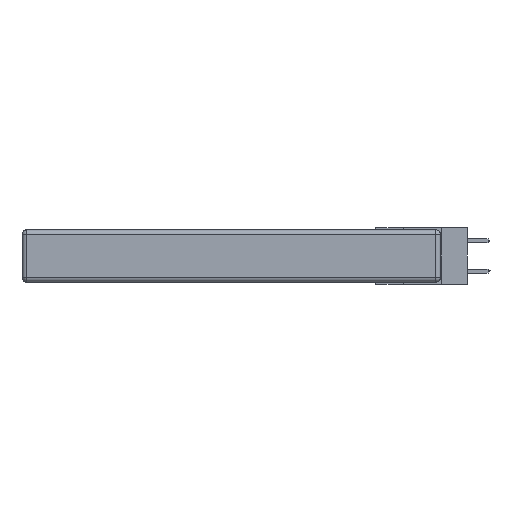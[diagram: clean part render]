
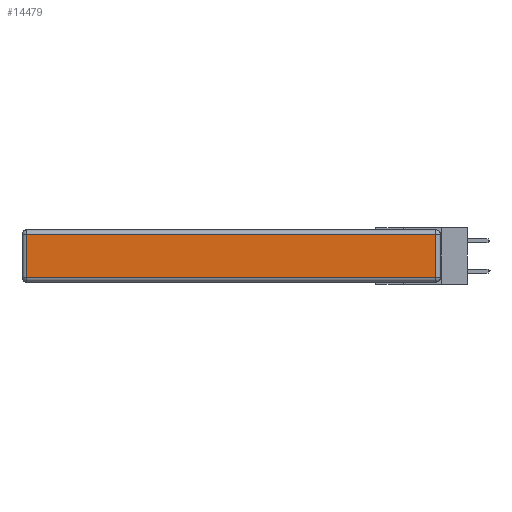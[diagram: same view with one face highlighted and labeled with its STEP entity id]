
A CAD part, left-side view. The second image highlights one B-rep face of the part: STEP entity #14479.
In plain terms, the highlighted planar face has unit normal (-1, 0, 0).
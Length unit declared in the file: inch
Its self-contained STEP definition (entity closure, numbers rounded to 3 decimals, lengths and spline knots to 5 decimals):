
#34 = CARTESIAN_POINT ( 'NONE',  ( 0., 2.72, -0.03 ) ) ;
#37 = DIRECTION ( 'NONE',  ( 0., 0., 1. ) ) ;
#346 = LINE ( 'NONE', #25565, #20899 ) ;
#1693 = ORIENTED_EDGE ( 'NONE', *, *, #17655, .T. ) ;
#5072 = VERTEX_POINT ( 'NONE', #11036 ) ;
#5687 = DIRECTION ( 'NONE',  ( 0., 1., 0. ) ) ;
#5783 = CARTESIAN_POINT ( 'NONE',  ( 0., 2.75, -0.03 ) ) ;
#7728 = CARTESIAN_POINT ( 'NONE',  ( 0., 0., -0.313 ) ) ;
#8910 = CARTESIAN_POINT ( 'NONE',  ( 0., 0.03, -0.343 ) ) ;
#9664 = DIRECTION ( 'NONE',  ( 0., -1., 0. ) ) ;
#10783 = PLANE ( 'NONE',  #12081 ) ;
#11036 = CARTESIAN_POINT ( 'NONE',  ( 0., 2.72, -0.313 ) ) ;
#11377 = VERTEX_POINT ( 'NONE', #17019 ) ;
#12081 = AXIS2_PLACEMENT_3D ( 'NONE', #24100, #13170, #37 ) ;
#12638 = VECTOR ( 'NONE', #9664, 39.37008 ) ;
#13128 = DIRECTION ( 'NONE',  ( 0., 0., 1. ) ) ;
#13170 = DIRECTION ( 'NONE',  ( -1., 0., 0. ) ) ;
#14479 = ADVANCED_FACE ( 'NONE', ( #22156 ), #10783, .T. ) ;
#14564 = ORIENTED_EDGE ( 'NONE', *, *, #26897, .T. ) ;
#15314 = EDGE_CURVE ( 'NONE', #11377, #20907, #17963, .T. ) ;
#15603 = VECTOR ( 'NONE', #5687, 39.37008 ) ;
#17019 = CARTESIAN_POINT ( 'NONE',  ( 0., 0.03, -0.03 ) ) ;
#17655 = EDGE_CURVE ( 'NONE', #20907, #5072, #346, .T. ) ;
#17670 = ORIENTED_EDGE ( 'NONE', *, *, #15314, .T. ) ;
#17800 = ORIENTED_EDGE ( 'NONE', *, *, #22877, .T. ) ;
#17963 = LINE ( 'NONE', #5783, #15603 ) ;
#18125 = LINE ( 'NONE', #8910, #22605 ) ;
#18182 = LINE ( 'NONE', #7728, #12638 ) ;
#19935 = VERTEX_POINT ( 'NONE', #27372 ) ;
#20899 = VECTOR ( 'NONE', #27961, 39.37008 ) ;
#20907 = VERTEX_POINT ( 'NONE', #34 ) ;
#22156 = FACE_OUTER_BOUND ( 'NONE', #26323, .T. ) ;
#22605 = VECTOR ( 'NONE', #13128, 39.37008 ) ;
#22877 = EDGE_CURVE ( 'NONE', #19935, #11377, #18125, .T. ) ;
#24100 = CARTESIAN_POINT ( 'NONE',  ( 0., 0., -0.343 ) ) ;
#25565 = CARTESIAN_POINT ( 'NONE',  ( 0., 2.72, -0.343 ) ) ;
#26323 = EDGE_LOOP ( 'NONE', ( #14564, #17800, #17670, #1693 ) ) ;
#26897 = EDGE_CURVE ( 'NONE', #5072, #19935, #18182, .T. ) ;
#27372 = CARTESIAN_POINT ( 'NONE',  ( 0., 0.03, -0.313 ) ) ;
#27961 = DIRECTION ( 'NONE',  ( 0., 0., -1. ) ) ;
